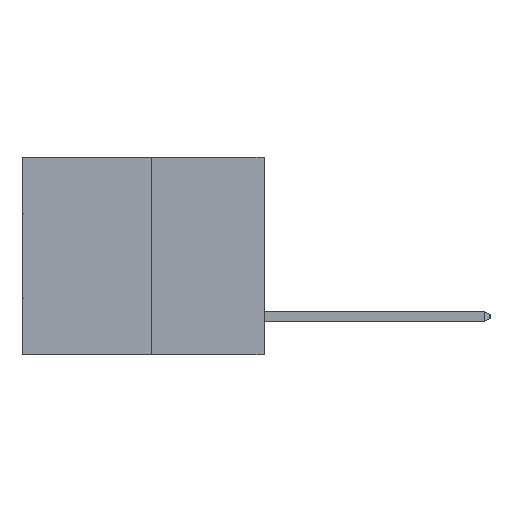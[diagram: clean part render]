
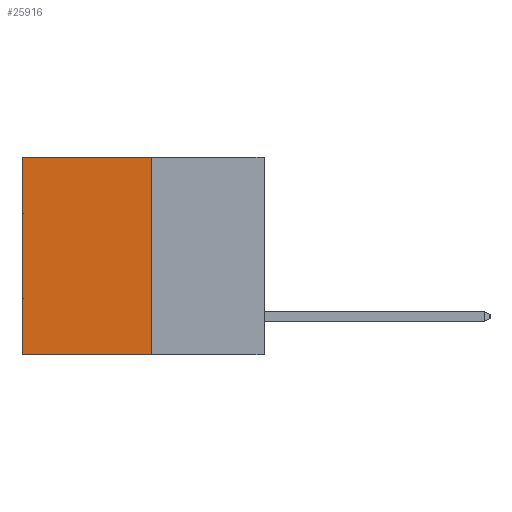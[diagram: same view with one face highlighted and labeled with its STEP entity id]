
A CAD part, left-side view. The second image highlights one B-rep face of the part: STEP entity #25916.
In plain terms, the highlighted planar face has unit normal (-1, 0, 0).
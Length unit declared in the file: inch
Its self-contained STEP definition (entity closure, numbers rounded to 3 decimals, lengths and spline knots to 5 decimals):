
#89 = DIRECTION ( 'NONE',  ( 0., 1., 0. ) ) ;
#178 = CARTESIAN_POINT ( 'NONE',  ( 0.3165, 0.28, -0.49 ) ) ;
#2236 = CARTESIAN_POINT ( 'NONE',  ( 0.3165, 0.6, 0. ) ) ;
#2955 = EDGE_CURVE ( 'NONE', #18670, #15440, #23461, .T. ) ;
#4071 = CARTESIAN_POINT ( 'NONE',  ( 0.3165, 0.6, -0.49 ) ) ;
#4209 = CARTESIAN_POINT ( 'NONE',  ( 0.3165, 0.28, -0.49 ) ) ;
#4255 = EDGE_CURVE ( 'NONE', #29698, #8280, #11429, .T. ) ;
#4965 = FACE_OUTER_BOUND ( 'NONE', #8125, .T. ) ;
#6228 = CARTESIAN_POINT ( 'NONE',  ( 0.3165, 0.28, -0.49 ) ) ;
#8125 = EDGE_LOOP ( 'NONE', ( #16980, #12267, #30623, #29692 ) ) ;
#8280 = VERTEX_POINT ( 'NONE', #2236 ) ;
#9097 = CARTESIAN_POINT ( 'NONE',  ( 0.3165, 0.6, -0.49 ) ) ;
#9581 = LINE ( 'NONE', #9097, #20470 ) ;
#10326 = VECTOR ( 'NONE', #89, 39.37008 ) ;
#11429 = LINE ( 'NONE', #22644, #30534 ) ;
#12238 = CARTESIAN_POINT ( 'NONE',  ( 0.3165, 0.28, -0.49 ) ) ;
#12267 = ORIENTED_EDGE ( 'NONE', *, *, #2955, .F. ) ;
#12375 = EDGE_CURVE ( 'NONE', #29698, #18670, #20066, .T. ) ;
#13952 = DIRECTION ( 'NONE',  ( 0., 0., -1. ) ) ;
#15440 = VERTEX_POINT ( 'NONE', #4071 ) ;
#15537 = DIRECTION ( 'NONE',  ( 1., 0., 0. ) ) ;
#15877 = EDGE_CURVE ( 'NONE', #8280, #15440, #9581, .T. ) ;
#16980 = ORIENTED_EDGE ( 'NONE', *, *, #15877, .T. ) ;
#18670 = VERTEX_POINT ( 'NONE', #178 ) ;
#20066 = LINE ( 'NONE', #4209, #30507 ) ;
#20470 = VECTOR ( 'NONE', #13952, 39.37008 ) ;
#21539 = AXIS2_PLACEMENT_3D ( 'NONE', #6228, #15537, #27775 ) ;
#22644 = CARTESIAN_POINT ( 'NONE',  ( 0.3165, 0.28, 0. ) ) ;
#22748 = DIRECTION ( 'NONE',  ( 0., 1., 0. ) ) ;
#23461 = LINE ( 'NONE', #12238, #10326 ) ;
#25110 = CARTESIAN_POINT ( 'NONE',  ( 0.3165, 0.28, 0. ) ) ;
#25146 = PLANE ( 'NONE',  #21539 ) ;
#25916 = ADVANCED_FACE ( 'NONE', ( #4965 ), #25146, .F. ) ;
#27775 = DIRECTION ( 'NONE',  ( 0., 0., -1. ) ) ;
#29692 = ORIENTED_EDGE ( 'NONE', *, *, #4255, .T. ) ;
#29698 = VERTEX_POINT ( 'NONE', #25110 ) ;
#30507 = VECTOR ( 'NONE', #30727, 39.37008 ) ;
#30534 = VECTOR ( 'NONE', #22748, 39.37008 ) ;
#30623 = ORIENTED_EDGE ( 'NONE', *, *, #12375, .F. ) ;
#30727 = DIRECTION ( 'NONE',  ( 0., 0., -1. ) ) ;
